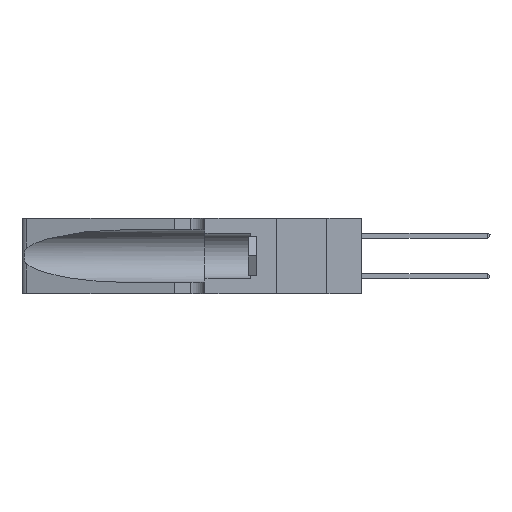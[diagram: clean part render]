
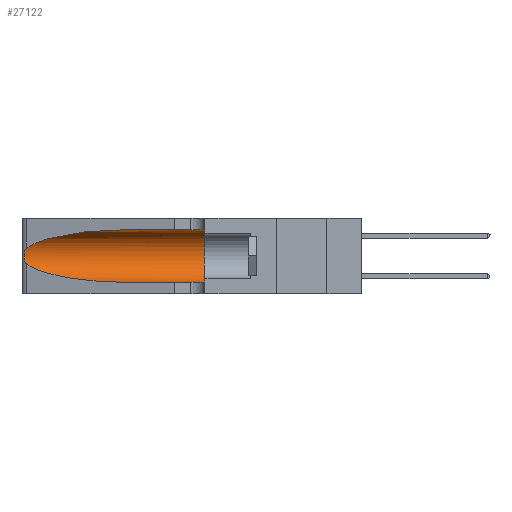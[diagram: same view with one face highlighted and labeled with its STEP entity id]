
A CAD part, left-side view. The second image highlights one B-rep face of the part: STEP entity #27122.
In plain terms, the highlighted cylindrical face has radius 3.308 mm (diameter 6.617 mm), a partial arc.
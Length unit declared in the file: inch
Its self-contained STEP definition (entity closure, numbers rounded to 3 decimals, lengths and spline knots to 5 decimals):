
#90 = DIRECTION ( 'NONE',  ( 0., -1., 0. ) ) ;
#656 = EDGE_CURVE ( 'NONE', #14309, #26448, #40594, .T. ) ;
#898 = DIRECTION ( 'NONE',  ( 0., -1., 0. ) ) ;
#1999 = CARTESIAN_POINT ( 'NONE',  ( 0.25555, 1.22994, 0.2215 ) ) ;
#2355 = CARTESIAN_POINT ( 'NONE',  ( 0.25487, 1.22718, 0.22369 ) ) ;
#2767 = CARTESIAN_POINT ( 'NONE',  ( 0.2373, 1.15595, 0.28018 ) ) ;
#3874 = DIRECTION ( 'NONE',  ( 0., 1., 0. ) ) ;
#3899 = CARTESIAN_POINT ( 'NONE',  ( 0.18966, 0.96281, 0.05475 ) ) ;
#5336 = CARTESIAN_POINT ( 'NONE',  ( 0.25787, 1.23484, 0.2124 ) ) ;
#5391 = AXIS2_PLACEMENT_3D ( 'NONE', #23531, #3874, #26812 ) ;
#6405 = VERTEX_POINT ( 'NONE', #15699 ) ;
#7048 = VERTEX_POINT ( 'NONE', #21912 ) ;
#7249 = ORIENTED_EDGE ( 'NONE', *, *, #21651, .F. ) ;
#8389 = EDGE_CURVE ( 'NONE', #6405, #26528, #33482, .T. ) ;
#8672 = CARTESIAN_POINT ( 'NONE',  ( 0.26018, 1.23835, 0.19895 ) ) ;
#10127 = EDGE_CURVE ( 'NONE', #14309, #40948, #25893, .T. ) ;
#11083 = CARTESIAN_POINT ( 'NONE',  ( 0.1305, 0.72297, 0.05475 ) ) ;
#11563 = ORIENTED_EDGE ( 'NONE', *, *, #8389, .T. ) ;
#11989 = CARTESIAN_POINT ( 'NONE',  ( 0.26075, 1.23896, 0.178 ) ) ;
#13396 = CYLINDRICAL_SURFACE ( 'NONE', #28844, 0.13025 ) ;
#14045 = DIRECTION ( 'NONE',  ( 0., 0., -1. ) ) ;
#14309 = VERTEX_POINT ( 'NONE', #39195 ) ;
#15201 = B_SPLINE_CURVE_WITH_KNOTS ( 'NONE', 3,
 ( #41234, #1999, #24961, #5336, #28223, #8672, #31530, #11989, #34801, #15288, #38086, #18537, #41369, #21818 ),
 .UNSPECIFIED., .F., .F.,
 ( 4, 2, 2, 2, 2, 2, 4 ),
 ( 0., 0.00027, 0.00053, 0.00107, 0.0016, 0.00187, 0.00214 ),
 .UNSPECIFIED. ) ;
#15279 = CARTESIAN_POINT ( 'NONE',  ( 0.1305, 0.35, 0.31525 ) ) ;
#15288 = CARTESIAN_POINT ( 'NONE',  ( 0.25856, 1.23593, 0.16098 ) ) ;
#15699 = CARTESIAN_POINT ( 'NONE',  ( 0.25487, 1.22718, 0.14631 ) ) ;
#17620 = ORIENTED_EDGE ( 'NONE', *, *, #37380, .T. ) ;
#18215 = LINE ( 'NONE', #29536, #42199 ) ;
#18537 = CARTESIAN_POINT ( 'NONE',  ( 0.25639, 1.23186, 0.15144 ) ) ;
#19161 = CARTESIAN_POINT ( 'NONE',  ( 0.18966, 0.96281, 0.31525 ) ) ;
#19433 = CIRCLE ( 'NONE', #5391, 0.13025 ) ;
#20268 = CARTESIAN_POINT ( 'NONE',  ( 0.25487, 1.22718, 0.14631 ) ) ;
#21651 = EDGE_CURVE ( 'NONE', #26448, #7048, #19433, .T. ) ;
#21818 = CARTESIAN_POINT ( 'NONE',  ( 0.25487, 1.22718, 0.14631 ) ) ;
#21912 = CARTESIAN_POINT ( 'NONE',  ( 0.1305, 0.35, 0.05475 ) ) ;
#23248 = VECTOR ( 'NONE', #90, 39.37008 ) ;
#23531 = CARTESIAN_POINT ( 'NONE',  ( 0.1305, 0.35, 0.185 ) ) ;
#23557 = CARTESIAN_POINT ( 'NONE',  ( 0.2373, 1.15595, 0.08982 ) ) ;
#24961 = CARTESIAN_POINT ( 'NONE',  ( 0.25639, 1.23184, 0.21858 ) ) ;
#25722 = CARTESIAN_POINT ( 'NONE',  ( 0.1305, 0.72297, 0.31525 ) ) ;
#25893 =( BOUNDED_CURVE ( )  B_SPLINE_CURVE ( 3, ( #25722, #19161, #2767, #28990 ),
 .UNSPECIFIED., .F., .T. ) 
 B_SPLINE_CURVE_WITH_KNOTS ( ( 4, 4 ),
 ( 1.5708, 2.84003 ),
 .UNSPECIFIED. ) 
 CURVE ( )  GEOMETRIC_REPRESENTATION_ITEM ( )  RATIONAL_B_SPLINE_CURVE ( ( 1., 0.87, 0.87, 1. ) ) 
 REPRESENTATION_ITEM ( '' )  );
#26448 = VERTEX_POINT ( 'NONE', #15279 ) ;
#26528 = VERTEX_POINT ( 'NONE', #11083 ) ;
#26812 = DIRECTION ( 'NONE',  ( 0., 0., 1. ) ) ;
#26832 = CARTESIAN_POINT ( 'NONE',  ( 0.1305, 0.72297, 0.05475 ) ) ;
#27122 = ADVANCED_FACE ( 'NONE', ( #31771 ), #13396, .F. ) ;
#28223 = CARTESIAN_POINT ( 'NONE',  ( 0.25854, 1.2359, 0.20912 ) ) ;
#28844 = AXIS2_PLACEMENT_3D ( 'NONE', #40133, #898, #14045 ) ;
#28990 = CARTESIAN_POINT ( 'NONE',  ( 0.25487, 1.22718, 0.22369 ) ) ;
#29491 = CARTESIAN_POINT ( 'NONE',  ( 0.1305, 1.61858, 0.31525 ) ) ;
#29536 = CARTESIAN_POINT ( 'NONE',  ( 0.1305, 1.61858, 0.05475 ) ) ;
#31530 = CARTESIAN_POINT ( 'NONE',  ( 0.26075, 1.23896, 0.19203 ) ) ;
#31771 = FACE_OUTER_BOUND ( 'NONE', #33992, .T. ) ;
#32065 = ORIENTED_EDGE ( 'NONE', *, *, #39712, .T. ) ;
#32975 = DIRECTION ( 'NONE',  ( 0., -1., 0. ) ) ;
#33482 =( BOUNDED_CURVE ( )  B_SPLINE_CURVE ( 3, ( #20268, #23557, #3899, #26832 ),
 .UNSPECIFIED., .F., .F. ) 
 B_SPLINE_CURVE_WITH_KNOTS ( ( 4, 4 ),
 ( 3.44316, 4.71239 ),
 .UNSPECIFIED. ) 
 CURVE ( )  GEOMETRIC_REPRESENTATION_ITEM ( )  RATIONAL_B_SPLINE_CURVE ( ( 1., 0.87, 0.87, 1. ) ) 
 REPRESENTATION_ITEM ( '' )  );
#33992 = EDGE_LOOP ( 'NONE', ( #39924, #32065, #11563, #17620, #7249, #41030 ) ) ;
#34801 = CARTESIAN_POINT ( 'NONE',  ( 0.26017, 1.23833, 0.17102 ) ) ;
#37380 = EDGE_CURVE ( 'NONE', #26528, #7048, #18215, .T. ) ;
#38086 = CARTESIAN_POINT ( 'NONE',  ( 0.25789, 1.23486, 0.15765 ) ) ;
#39195 = CARTESIAN_POINT ( 'NONE',  ( 0.1305, 0.72297, 0.31525 ) ) ;
#39712 = EDGE_CURVE ( 'NONE', #40948, #6405, #15201, .T. ) ;
#39924 = ORIENTED_EDGE ( 'NONE', *, *, #10127, .T. ) ;
#40133 = CARTESIAN_POINT ( 'NONE',  ( 0.1305, 1.61858, 0.185 ) ) ;
#40594 = LINE ( 'NONE', #29491, #23248 ) ;
#40948 = VERTEX_POINT ( 'NONE', #2355 ) ;
#41030 = ORIENTED_EDGE ( 'NONE', *, *, #656, .F. ) ;
#41234 = CARTESIAN_POINT ( 'NONE',  ( 0.25487, 1.22718, 0.22369 ) ) ;
#41369 = CARTESIAN_POINT ( 'NONE',  ( 0.25555, 1.22993, 0.14849 ) ) ;
#42199 = VECTOR ( 'NONE', #32975, 39.37008 ) ;
